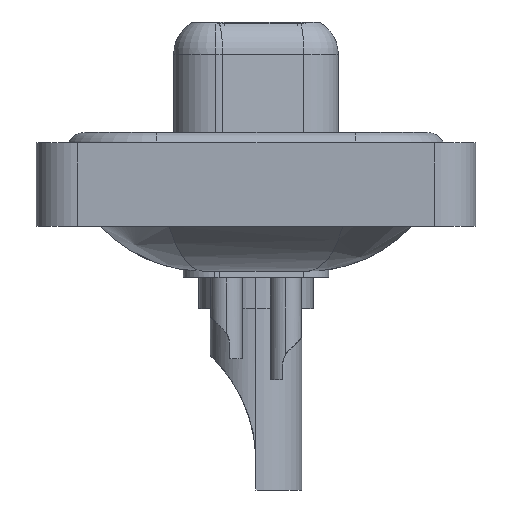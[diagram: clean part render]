
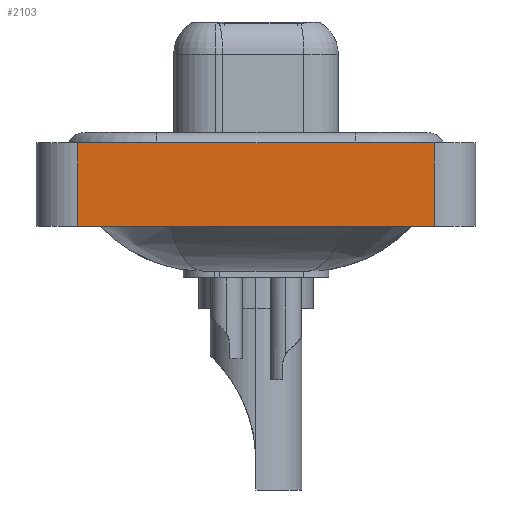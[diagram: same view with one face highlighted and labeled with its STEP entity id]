
A CAD part, left-side view. The second image highlights one B-rep face of the part: STEP entity #2103.
In plain terms, the highlighted planar face has unit normal (-1, 0, 0).
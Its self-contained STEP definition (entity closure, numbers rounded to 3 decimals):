
#242 = EDGE_CURVE ( 'NONE', #1517, #879, #11291, .T. ) ;
#406 = CARTESIAN_POINT ( 'NONE',  ( -7.3, -8.55, -3.6 ) ) ;
#879 = VERTEX_POINT ( 'NONE', #3786 ) ;
#1517 = VERTEX_POINT ( 'NONE', #18234 ) ;
#1608 = EDGE_LOOP ( 'NONE', ( #21487, #17792, #20869, #20555 ) ) ;
#2024 = CARTESIAN_POINT ( 'NONE',  ( -7.3, 8.55, -3.6 ) ) ;
#2103 = ADVANCED_FACE ( 'NONE', ( #20679 ), #3474, .T. ) ;
#2265 = EDGE_CURVE ( 'NONE', #879, #21274, #3912, .T. ) ;
#3474 = PLANE ( 'NONE',  #13937 ) ;
#3786 = CARTESIAN_POINT ( 'NONE',  ( -7.3, -8.55, -3.6 ) ) ;
#3912 = LINE ( 'NONE', #406, #20461 ) ;
#4306 = LINE ( 'NONE', #11177, #6843 ) ;
#4341 = VECTOR ( 'NONE', #5535, 1000. ) ;
#5535 = DIRECTION ( 'NONE',  ( 0., 0., 1. ) ) ;
#5841 = DIRECTION ( 'NONE',  ( 0., 0., 1. ) ) ;
#6843 = VECTOR ( 'NONE', #18130, 1000. ) ;
#6980 = CARTESIAN_POINT ( 'NONE',  ( -7.3, -8.55, -3.6 ) ) ;
#11060 = DIRECTION ( 'NONE',  ( 0., -1., 0. ) ) ;
#11177 = CARTESIAN_POINT ( 'NONE',  ( -7.3, -8.55, 0.4 ) ) ;
#11291 = LINE ( 'NONE', #18233, #12189 ) ;
#12189 = VECTOR ( 'NONE', #11060, 1000. ) ;
#13937 = AXIS2_PLACEMENT_3D ( 'NONE', #6980, #17410, #22280 ) ;
#14114 = EDGE_CURVE ( 'NONE', #14858, #21274, #4306, .T. ) ;
#14858 = VERTEX_POINT ( 'NONE', #17415 ) ;
#17410 = DIRECTION ( 'NONE',  ( -1., 0., 0. ) ) ;
#17415 = CARTESIAN_POINT ( 'NONE',  ( -7.3, 8.55, 0.4 ) ) ;
#17792 = ORIENTED_EDGE ( 'NONE', *, *, #14114, .F. ) ;
#18130 = DIRECTION ( 'NONE',  ( 0., -1., 0. ) ) ;
#18233 = CARTESIAN_POINT ( 'NONE',  ( -7.3, -8.55, -3.6 ) ) ;
#18234 = CARTESIAN_POINT ( 'NONE',  ( -7.3, 8.55, -3.6 ) ) ;
#19216 = EDGE_CURVE ( 'NONE', #1517, #14858, #20811, .T. ) ;
#20461 = VECTOR ( 'NONE', #5841, 1000. ) ;
#20555 = ORIENTED_EDGE ( 'NONE', *, *, #242, .T. ) ;
#20679 = FACE_OUTER_BOUND ( 'NONE', #1608, .T. ) ;
#20811 = LINE ( 'NONE', #2024, #4341 ) ;
#20866 = CARTESIAN_POINT ( 'NONE',  ( -7.3, -8.55, 0.4 ) ) ;
#20869 = ORIENTED_EDGE ( 'NONE', *, *, #19216, .F. ) ;
#21274 = VERTEX_POINT ( 'NONE', #20866 ) ;
#21487 = ORIENTED_EDGE ( 'NONE', *, *, #2265, .T. ) ;
#22280 = DIRECTION ( 'NONE',  ( 0., 0., 1. ) ) ;
